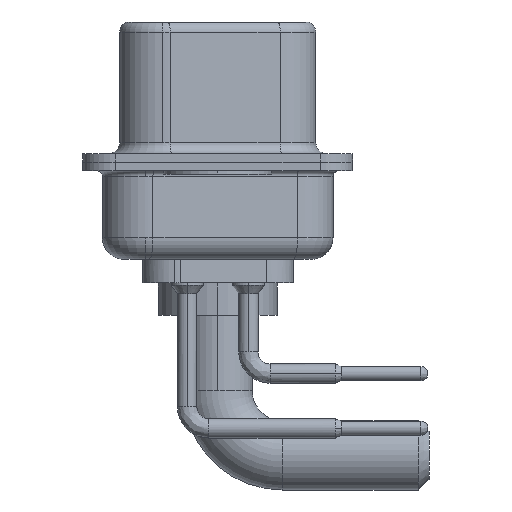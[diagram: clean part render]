
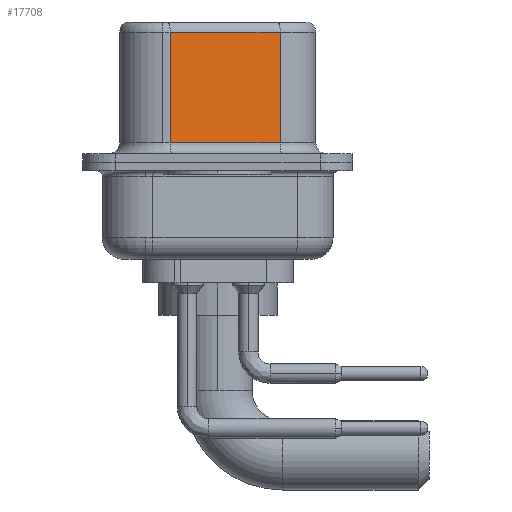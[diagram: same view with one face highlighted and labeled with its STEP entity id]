
A CAD part, left-side view. The second image highlights one B-rep face of the part: STEP entity #17708.
In plain terms, the highlighted planar face has unit normal (-0.985, -0.174, 0).
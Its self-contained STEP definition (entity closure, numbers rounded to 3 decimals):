
#740 = DIRECTION ( 'NONE',  ( 0., 0., -1. ) ) ;
#854 = DIRECTION ( 'NONE',  ( -0.174, 0.985, 0. ) ) ;
#4520 = CARTESIAN_POINT ( 'NONE',  ( 4.58, -2.897, 6.52 ) ) ;
#5320 = EDGE_LOOP ( 'NONE', ( #12353, #5912, #8867, #6171 ) ) ;
#5912 = ORIENTED_EDGE ( 'NONE', *, *, #22976, .T. ) ;
#6171 = ORIENTED_EDGE ( 'NONE', *, *, #8016, .T. ) ;
#6349 = CARTESIAN_POINT ( 'NONE',  ( 3.68, 2.203, 6.52 ) ) ;
#6383 = DIRECTION ( 'NONE',  ( -0.174, 0.985, 0. ) ) ;
#7086 = CARTESIAN_POINT ( 'NONE',  ( 3.68, 2.203, 6.02 ) ) ;
#7485 = DIRECTION ( 'NONE',  ( 0.174, -0.985, 0. ) ) ;
#8016 = EDGE_CURVE ( 'NONE', #9263, #13392, #13337, .T. ) ;
#8867 = ORIENTED_EDGE ( 'NONE', *, *, #21654, .T. ) ;
#9263 = VERTEX_POINT ( 'NONE', #11158 ) ;
#10392 = LINE ( 'NONE', #12117, #12756 ) ;
#11158 = CARTESIAN_POINT ( 'NONE',  ( 3.68, 2.203, 0.9 ) ) ;
#12117 = CARTESIAN_POINT ( 'NONE',  ( 4.58, -2.897, 6.02 ) ) ;
#12353 = ORIENTED_EDGE ( 'NONE', *, *, #20274, .F. ) ;
#12756 = VECTOR ( 'NONE', #6383, 1000. ) ;
#13291 = CARTESIAN_POINT ( 'NONE',  ( 4.58, -2.897, 6.52 ) ) ;
#13337 = LINE ( 'NONE', #16856, #16655 ) ;
#13392 = VERTEX_POINT ( 'NONE', #20848 ) ;
#14629 = VECTOR ( 'NONE', #21317, 1000. ) ;
#15117 = LINE ( 'NONE', #13291, #21612 ) ;
#15605 = LINE ( 'NONE', #6349, #14629 ) ;
#15620 = CARTESIAN_POINT ( 'NONE',  ( 4.58, -2.897, 6.02 ) ) ;
#16655 = VECTOR ( 'NONE', #7485, 1000. ) ;
#16856 = CARTESIAN_POINT ( 'NONE',  ( 4.58, -2.897, 0.9 ) ) ;
#17280 = VERTEX_POINT ( 'NONE', #15620 ) ;
#17708 = ADVANCED_FACE ( 'NONE', ( #21186 ), #20946, .F. ) ;
#19144 = DIRECTION ( 'NONE',  ( 0.985, 0.174, 0. ) ) ;
#20110 = VERTEX_POINT ( 'NONE', #7086 ) ;
#20274 = EDGE_CURVE ( 'NONE', #17280, #13392, #15117, .T. ) ;
#20848 = CARTESIAN_POINT ( 'NONE',  ( 4.58, -2.897, 0.9 ) ) ;
#20946 = PLANE ( 'NONE',  #22347 ) ;
#21186 = FACE_OUTER_BOUND ( 'NONE', #5320, .T. ) ;
#21317 = DIRECTION ( 'NONE',  ( 0., 0., -1. ) ) ;
#21612 = VECTOR ( 'NONE', #740, 1000. ) ;
#21654 = EDGE_CURVE ( 'NONE', #20110, #9263, #15605, .T. ) ;
#22347 = AXIS2_PLACEMENT_3D ( 'NONE', #4520, #19144, #854 ) ;
#22976 = EDGE_CURVE ( 'NONE', #17280, #20110, #10392, .T. ) ;
